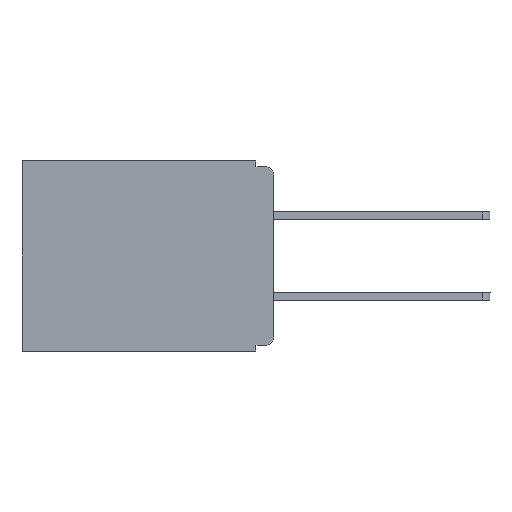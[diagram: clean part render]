
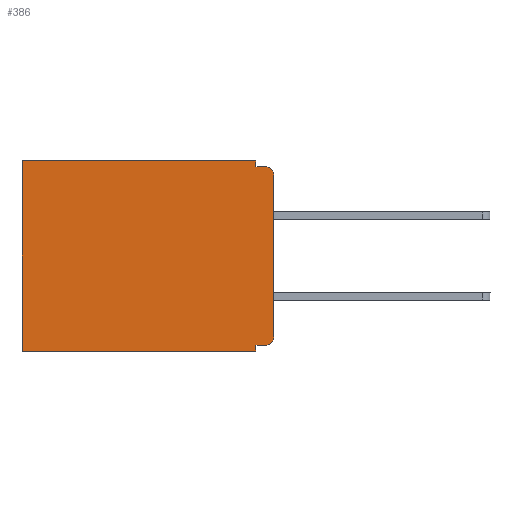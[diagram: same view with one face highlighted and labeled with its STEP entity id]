
A CAD part, left-side view. The second image highlights one B-rep face of the part: STEP entity #386.
In plain terms, the highlighted planar face has unit normal (-1, 0, 0).
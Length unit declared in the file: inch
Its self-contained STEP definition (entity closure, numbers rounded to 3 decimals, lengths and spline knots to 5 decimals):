
#358 = VECTOR ( 'NONE', #5700, 39.37008 ) ;
#386 = ADVANCED_FACE ( 'NONE', ( #6312 ), #9788, .F. ) ;
#407 = CIRCLE ( 'NONE', #3867, 0.015 ) ;
#410 = VERTEX_POINT ( 'NONE', #3166 ) ;
#477 = EDGE_CURVE ( 'NONE', #4897, #5716, #6840, .T. ) ;
#649 = VECTOR ( 'NONE', #890, 39.37008 ) ;
#682 = DIRECTION ( 'NONE',  ( 0., 0., -1. ) ) ;
#750 = LINE ( 'NONE', #6791, #6163 ) ;
#890 = DIRECTION ( 'NONE',  ( 0., 0., -1. ) ) ;
#1044 = EDGE_CURVE ( 'NONE', #4897, #1997, #1558, .T. ) ;
#1170 = EDGE_CURVE ( 'NONE', #5465, #5713, #2826, .T. ) ;
#1192 = ORIENTED_EDGE ( 'NONE', *, *, #3423, .F. ) ;
#1558 = LINE ( 'NONE', #7279, #6728 ) ;
#1657 = DIRECTION ( 'NONE',  ( 1., 0., 0. ) ) ;
#1692 = DIRECTION ( 'NONE',  ( 0., 0., -1. ) ) ;
#1729 = CARTESIAN_POINT ( 'NONE',  ( 0.3, 0., -0.33 ) ) ;
#1782 = AXIS2_PLACEMENT_3D ( 'NONE', #1797, #7036, #2903 ) ;
#1783 = CARTESIAN_POINT ( 'NONE',  ( 0.3, 0., -0.025 ) ) ;
#1794 = EDGE_CURVE ( 'NONE', #410, #8381, #7336, .T. ) ;
#1797 = CARTESIAN_POINT ( 'NONE',  ( 0.3, 0.015, -0.025 ) ) ;
#1997 = VERTEX_POINT ( 'NONE', #7386 ) ;
#2438 = VECTOR ( 'NONE', #6437, 39.37008 ) ;
#2510 = VERTEX_POINT ( 'NONE', #8584 ) ;
#2826 = LINE ( 'NONE', #4127, #649 ) ;
#2903 = DIRECTION ( 'NONE',  ( 0., 0., -1. ) ) ;
#3114 = EDGE_LOOP ( 'NONE', ( #8954, #5382, #8951, #6014, #8292, #9448, #1192, #3535, #7014, #9749 ) ) ;
#3151 = VECTOR ( 'NONE', #9248, 39.37008 ) ;
#3166 = CARTESIAN_POINT ( 'NONE',  ( 0.3, 0.437, 0. ) ) ;
#3423 = EDGE_CURVE ( 'NONE', #5713, #8381, #4961, .T. ) ;
#3535 = ORIENTED_EDGE ( 'NONE', *, *, #1170, .F. ) ;
#3585 = CARTESIAN_POINT ( 'NONE',  ( 0.3, 0.031, 0. ) ) ;
#3636 = DIRECTION ( 'NONE',  ( 0., 1., 0. ) ) ;
#3867 = AXIS2_PLACEMENT_3D ( 'NONE', #5425, #6273, #6311 ) ;
#4106 = EDGE_CURVE ( 'NONE', #2510, #9934, #8579, .T. ) ;
#4127 = CARTESIAN_POINT ( 'NONE',  ( 0.3, 0.031, -0.33 ) ) ;
#4248 = CARTESIAN_POINT ( 'NONE',  ( 0.3, 0.015, -0.32 ) ) ;
#4557 = AXIS2_PLACEMENT_3D ( 'NONE', #9106, #1657, #1692 ) ;
#4630 = CARTESIAN_POINT ( 'NONE',  ( 0.3, 0.437, -0.33 ) ) ;
#4793 = CARTESIAN_POINT ( 'NONE',  ( 0.3, 0.031, -0.32 ) ) ;
#4882 = DIRECTION ( 'NONE',  ( 0., -1., 0. ) ) ;
#4897 = VERTEX_POINT ( 'NONE', #1783 ) ;
#4948 = CARTESIAN_POINT ( 'NONE',  ( 0.3, 0., -0.01 ) ) ;
#4961 = LINE ( 'NONE', #1729, #3151 ) ;
#5227 = DIRECTION ( 'NONE',  ( 0., 0., -1. ) ) ;
#5382 = ORIENTED_EDGE ( 'NONE', *, *, #477, .T. ) ;
#5425 = CARTESIAN_POINT ( 'NONE',  ( 0.3, 0.015, -0.305 ) ) ;
#5465 = VERTEX_POINT ( 'NONE', #4793 ) ;
#5567 = CARTESIAN_POINT ( 'NONE',  ( 0.3, 0.437, -0.33 ) ) ;
#5700 = DIRECTION ( 'NONE',  ( 0., 1., 0. ) ) ;
#5710 = VECTOR ( 'NONE', #5227, 39.37008 ) ;
#5713 = VERTEX_POINT ( 'NONE', #6074 ) ;
#5716 = VERTEX_POINT ( 'NONE', #9335 ) ;
#5973 = EDGE_CURVE ( 'NONE', #9934, #5716, #9076, .T. ) ;
#6014 = ORIENTED_EDGE ( 'NONE', *, *, #4106, .F. ) ;
#6074 = CARTESIAN_POINT ( 'NONE',  ( 0.3, 0.031, -0.33 ) ) ;
#6163 = VECTOR ( 'NONE', #3636, 39.37008 ) ;
#6273 = DIRECTION ( 'NONE',  ( -1., 0., 0. ) ) ;
#6311 = DIRECTION ( 'NONE',  ( 0., 0., -1. ) ) ;
#6312 = FACE_OUTER_BOUND ( 'NONE', #3114, .T. ) ;
#6437 = DIRECTION ( 'NONE',  ( 0., 0., -1. ) ) ;
#6639 = VECTOR ( 'NONE', #4882, 39.37008 ) ;
#6728 = VECTOR ( 'NONE', #682, 39.37008 ) ;
#6791 = CARTESIAN_POINT ( 'NONE',  ( 0.3, 0., -0.32 ) ) ;
#6840 = CIRCLE ( 'NONE', #1782, 0.015 ) ;
#6911 = EDGE_CURVE ( 'NONE', #8801, #1997, #407, .T. ) ;
#7014 = ORIENTED_EDGE ( 'NONE', *, *, #8247, .F. ) ;
#7036 = DIRECTION ( 'NONE',  ( -1., 0., 0. ) ) ;
#7279 = CARTESIAN_POINT ( 'NONE',  ( 0.3, 0., -0.33 ) ) ;
#7336 = LINE ( 'NONE', #5567, #2438 ) ;
#7375 = CARTESIAN_POINT ( 'NONE',  ( 0.3, 0., 0. ) ) ;
#7386 = CARTESIAN_POINT ( 'NONE',  ( 0.3, 0., -0.305 ) ) ;
#8247 = EDGE_CURVE ( 'NONE', #8801, #5465, #750, .T. ) ;
#8292 = ORIENTED_EDGE ( 'NONE', *, *, #8641, .T. ) ;
#8360 = LINE ( 'NONE', #7375, #358 ) ;
#8381 = VERTEX_POINT ( 'NONE', #4630 ) ;
#8579 = LINE ( 'NONE', #3585, #5710 ) ;
#8584 = CARTESIAN_POINT ( 'NONE',  ( 0.3, 0.031, 0. ) ) ;
#8641 = EDGE_CURVE ( 'NONE', #2510, #410, #8360, .T. ) ;
#8801 = VERTEX_POINT ( 'NONE', #4248 ) ;
#8951 = ORIENTED_EDGE ( 'NONE', *, *, #5973, .F. ) ;
#8954 = ORIENTED_EDGE ( 'NONE', *, *, #1044, .F. ) ;
#9076 = LINE ( 'NONE', #4948, #6639 ) ;
#9106 = CARTESIAN_POINT ( 'NONE',  ( 0.3, 0., -0.33 ) ) ;
#9248 = DIRECTION ( 'NONE',  ( 0., 1., 0. ) ) ;
#9335 = CARTESIAN_POINT ( 'NONE',  ( 0.3, 0.015, -0.01 ) ) ;
#9448 = ORIENTED_EDGE ( 'NONE', *, *, #1794, .T. ) ;
#9749 = ORIENTED_EDGE ( 'NONE', *, *, #6911, .T. ) ;
#9788 = PLANE ( 'NONE',  #4557 ) ;
#9934 = VERTEX_POINT ( 'NONE', #10699 ) ;
#10699 = CARTESIAN_POINT ( 'NONE',  ( 0.3, 0.031, -0.01 ) ) ;
